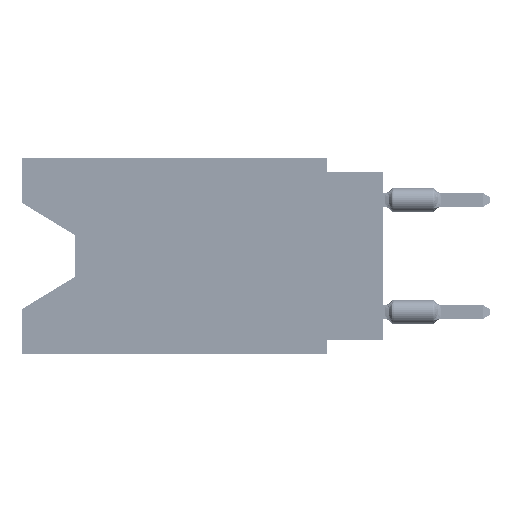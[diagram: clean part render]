
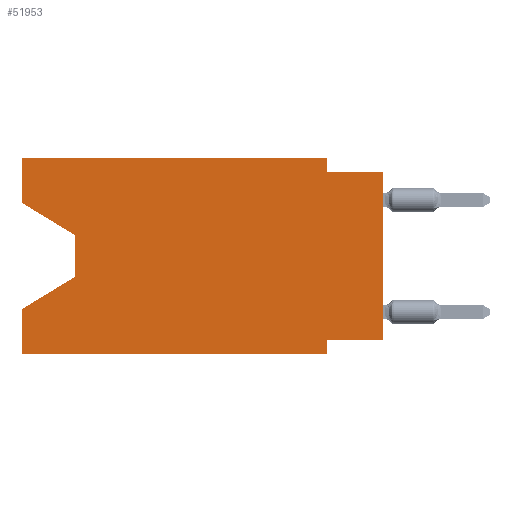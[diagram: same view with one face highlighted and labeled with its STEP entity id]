
A CAD part, left-side view. The second image highlights one B-rep face of the part: STEP entity #51953.
In plain terms, the highlighted planar face has unit normal (-1, 0, 0).
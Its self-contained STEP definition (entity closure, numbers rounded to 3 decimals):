
#187 = EDGE_CURVE ( 'NONE', #54515, #7736, #53673, .T. ) ;
#337 = CARTESIAN_POINT ( 'NONE',  ( 0., 2.54, 0. ) ) ;
#593 = FACE_OUTER_BOUND ( 'NONE', #21126, .T. ) ;
#1557 = CARTESIAN_POINT ( 'NONE',  ( 0., 16.383, -6.852 ) ) ;
#2699 = EDGE_CURVE ( 'NONE', #52868, #49029, #30171, .T. ) ;
#3339 = LINE ( 'NONE', #13506, #3406 ) ;
#3406 = VECTOR ( 'NONE', #46432, 1000. ) ;
#3893 = EDGE_CURVE ( 'NONE', #48624, #7736, #43560, .T. ) ;
#4792 = VECTOR ( 'NONE', #20908, 1000. ) ;
#4975 = EDGE_CURVE ( 'NONE', #35965, #50709, #23042, .T. ) ;
#5137 = LINE ( 'NONE', #42960, #4792 ) ;
#5810 = VERTEX_POINT ( 'NONE', #59682 ) ;
#6303 = ORIENTED_EDGE ( 'NONE', *, *, #52517, .F. ) ;
#7736 = VERTEX_POINT ( 'NONE', #27198 ) ;
#10232 = CARTESIAN_POINT ( 'NONE',  ( 0., 2.54, -8.89 ) ) ;
#11027 = CARTESIAN_POINT ( 'NONE',  ( 0., 0., -8.255 ) ) ;
#11097 = DIRECTION ( 'NONE',  ( 0., 0., -1. ) ) ;
#13506 = CARTESIAN_POINT ( 'NONE',  ( 0., 13.97, -5.385 ) ) ;
#13947 = VECTOR ( 'NONE', #26018, 1000. ) ;
#14027 = VERTEX_POINT ( 'NONE', #43040 ) ;
#16237 = ORIENTED_EDGE ( 'NONE', *, *, #56421, .T. ) ;
#16873 = CARTESIAN_POINT ( 'NONE',  ( 0., 16.383, -8.89 ) ) ;
#17910 = DIRECTION ( 'NONE',  ( 0., 1., 0. ) ) ;
#18069 = VECTOR ( 'NONE', #36537, 1000. ) ;
#18452 = ORIENTED_EDGE ( 'NONE', *, *, #62868, .F. ) ;
#18470 = ORIENTED_EDGE ( 'NONE', *, *, #53321, .F. ) ;
#19856 = ORIENTED_EDGE ( 'NONE', *, *, #67986, .F. ) ;
#20434 = ORIENTED_EDGE ( 'NONE', *, *, #51318, .T. ) ;
#20674 = DIRECTION ( 'NONE',  ( 0., 0., -1. ) ) ;
#20908 = DIRECTION ( 'NONE',  ( 0., -1., 0. ) ) ;
#21126 = EDGE_LOOP ( 'NONE', ( #16237, #20434, #68234, #19856, #44137, #59958, #6303, #37620, #18452, #46579, #18470, #36506 ) ) ;
#21467 = VERTEX_POINT ( 'NONE', #1557 ) ;
#21972 = LINE ( 'NONE', #43331, #60844 ) ;
#22704 = CARTESIAN_POINT ( 'NONE',  ( 0., 16.383, 0. ) ) ;
#23042 = LINE ( 'NONE', #22704, #53368 ) ;
#24763 = VECTOR ( 'NONE', #52727, 1000. ) ;
#26018 = DIRECTION ( 'NONE',  ( 0., 0., -1. ) ) ;
#27198 = CARTESIAN_POINT ( 'NONE',  ( 0., 2.54, -8.89 ) ) ;
#29104 = DIRECTION ( 'NONE',  ( 0., 0., 1. ) ) ;
#29494 = VECTOR ( 'NONE', #20674, 1000. ) ;
#29543 = AXIS2_PLACEMENT_3D ( 'NONE', #59089, #63636, #11097 ) ;
#30171 = LINE ( 'NONE', #51197, #62056 ) ;
#30578 = CARTESIAN_POINT ( 'NONE',  ( 0., 16.383, -2.038 ) ) ;
#31255 = CARTESIAN_POINT ( 'NONE',  ( 0., 16.383, -2.038 ) ) ;
#31789 = CARTESIAN_POINT ( 'NONE',  ( 0., 2.54, -8.255 ) ) ;
#32898 = CARTESIAN_POINT ( 'NONE',  ( 0., 2.54, -0.635 ) ) ;
#33057 = DIRECTION ( 'NONE',  ( 0., -1., 0. ) ) ;
#34162 = VECTOR ( 'NONE', #33057, 1000. ) ;
#34364 = LINE ( 'NONE', #55736, #51093 ) ;
#35965 = VERTEX_POINT ( 'NONE', #31255 ) ;
#36506 = ORIENTED_EDGE ( 'NONE', *, *, #4975, .F. ) ;
#36537 = DIRECTION ( 'NONE',  ( 0., -0.855, -0.519 ) ) ;
#37620 = ORIENTED_EDGE ( 'NONE', *, *, #42536, .T. ) ;
#38019 = CARTESIAN_POINT ( 'NONE',  ( 0., 0., 0. ) ) ;
#40646 = CARTESIAN_POINT ( 'NONE',  ( 0., 0., -8.255 ) ) ;
#41150 = EDGE_CURVE ( 'NONE', #5810, #21467, #3339, .T. ) ;
#42279 = PLANE ( 'NONE',  #29543 ) ;
#42536 = EDGE_CURVE ( 'NONE', #53682, #14027, #48530, .T. ) ;
#42960 = CARTESIAN_POINT ( 'NONE',  ( 0., 0., -0.635 ) ) ;
#43040 = CARTESIAN_POINT ( 'NONE',  ( 0., 0., -0.635 ) ) ;
#43331 = CARTESIAN_POINT ( 'NONE',  ( 0., 16.383, 0. ) ) ;
#43560 = LINE ( 'NONE', #59684, #34162 ) ;
#44137 = ORIENTED_EDGE ( 'NONE', *, *, #3893, .T. ) ;
#46003 = LINE ( 'NONE', #30578, #18069 ) ;
#46243 = CARTESIAN_POINT ( 'NONE',  ( 0., 13.97, -3.505 ) ) ;
#46351 = VERTEX_POINT ( 'NONE', #65920 ) ;
#46432 = DIRECTION ( 'NONE',  ( 0., 0.855, -0.519 ) ) ;
#46579 = ORIENTED_EDGE ( 'NONE', *, *, #2699, .F. ) ;
#48507 = VECTOR ( 'NONE', #17910, 1000. ) ;
#48530 = LINE ( 'NONE', #38019, #24763 ) ;
#48624 = VERTEX_POINT ( 'NONE', #16873 ) ;
#48637 = DIRECTION ( 'NONE',  ( 0., 0., 1. ) ) ;
#49029 = VERTEX_POINT ( 'NONE', #32898 ) ;
#49783 = LINE ( 'NONE', #40646, #48507 ) ;
#50709 = VERTEX_POINT ( 'NONE', #54432 ) ;
#51093 = VECTOR ( 'NONE', #29104, 1000. ) ;
#51197 = CARTESIAN_POINT ( 'NONE',  ( 0., 2.54, 0. ) ) ;
#51318 = EDGE_CURVE ( 'NONE', #46351, #5810, #56760, .T. ) ;
#51953 = ADVANCED_FACE ( 'NONE', ( #593 ), #42279, .F. ) ;
#52517 = EDGE_CURVE ( 'NONE', #53682, #54515, #49783, .T. ) ;
#52727 = DIRECTION ( 'NONE',  ( 0., 0., 1. ) ) ;
#52868 = VERTEX_POINT ( 'NONE', #337 ) ;
#53321 = EDGE_CURVE ( 'NONE', #50709, #52868, #21972, .T. ) ;
#53368 = VECTOR ( 'NONE', #48637, 1000. ) ;
#53673 = LINE ( 'NONE', #10232, #13947 ) ;
#53682 = VERTEX_POINT ( 'NONE', #11027 ) ;
#54432 = CARTESIAN_POINT ( 'NONE',  ( 0., 16.383, 0. ) ) ;
#54515 = VERTEX_POINT ( 'NONE', #31789 ) ;
#55736 = CARTESIAN_POINT ( 'NONE',  ( 0., 16.383, 0. ) ) ;
#55778 = DIRECTION ( 'NONE',  ( 0., 0., -1. ) ) ;
#56421 = EDGE_CURVE ( 'NONE', #35965, #46351, #46003, .T. ) ;
#56760 = LINE ( 'NONE', #46243, #29494 ) ;
#59089 = CARTESIAN_POINT ( 'NONE',  ( 0., 16.383, 0. ) ) ;
#59682 = CARTESIAN_POINT ( 'NONE',  ( 0., 13.97, -5.385 ) ) ;
#59684 = CARTESIAN_POINT ( 'NONE',  ( 0., 16.383, -8.89 ) ) ;
#59958 = ORIENTED_EDGE ( 'NONE', *, *, #187, .F. ) ;
#60844 = VECTOR ( 'NONE', #64689, 1000. ) ;
#62056 = VECTOR ( 'NONE', #55778, 1000. ) ;
#62868 = EDGE_CURVE ( 'NONE', #49029, #14027, #5137, .T. ) ;
#63636 = DIRECTION ( 'NONE',  ( 1., 0., 0. ) ) ;
#64689 = DIRECTION ( 'NONE',  ( 0., -1., 0. ) ) ;
#65920 = CARTESIAN_POINT ( 'NONE',  ( 0., 13.97, -3.505 ) ) ;
#67986 = EDGE_CURVE ( 'NONE', #48624, #21467, #34364, .T. ) ;
#68234 = ORIENTED_EDGE ( 'NONE', *, *, #41150, .T. ) ;
